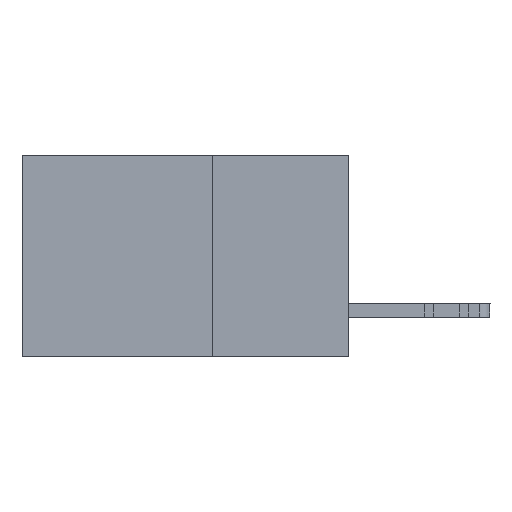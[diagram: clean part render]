
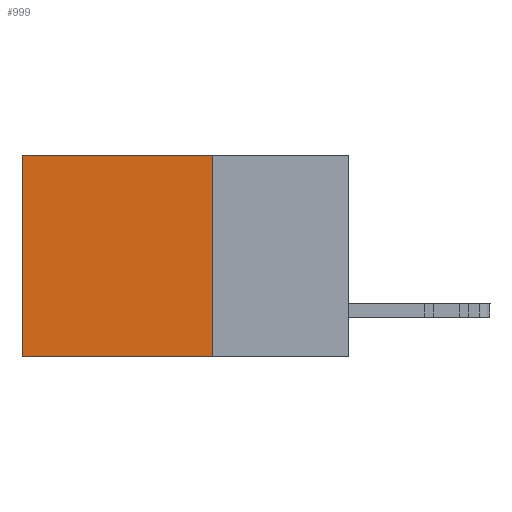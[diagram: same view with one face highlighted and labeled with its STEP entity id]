
A CAD part, left-side view. The second image highlights one B-rep face of the part: STEP entity #999.
In plain terms, the highlighted planar face has unit normal (-1, 0, 0).
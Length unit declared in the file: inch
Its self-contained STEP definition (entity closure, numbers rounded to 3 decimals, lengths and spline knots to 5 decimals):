
#294 = CARTESIAN_POINT ( 'NONE',  ( 0.2615, 0.25, -0.37 ) ) ;
#839 = DIRECTION ( 'NONE',  ( 0., 1., 0. ) ) ;
#999 = ADVANCED_FACE ( 'NONE', ( #12990 ), #22394, .F. ) ;
#1249 = VERTEX_POINT ( 'NONE', #13053 ) ;
#1746 = ORIENTED_EDGE ( 'NONE', *, *, #7309, .F. ) ;
#2405 = LINE ( 'NONE', #9855, #22892 ) ;
#4763 = CARTESIAN_POINT ( 'NONE',  ( 0.2615, 0.6, -0.37 ) ) ;
#5601 = VECTOR ( 'NONE', #7754, 39.37008 ) ;
#6305 = VERTEX_POINT ( 'NONE', #11732 ) ;
#7187 = CARTESIAN_POINT ( 'NONE',  ( 0.2615, 0.25, 0. ) ) ;
#7309 = EDGE_CURVE ( 'NONE', #17852, #19011, #2405, .T. ) ;
#7754 = DIRECTION ( 'NONE',  ( 0., 1., 0. ) ) ;
#8669 = AXIS2_PLACEMENT_3D ( 'NONE', #20450, #22514, #18620 ) ;
#9855 = CARTESIAN_POINT ( 'NONE',  ( 0.2615, 0.25, -0.37 ) ) ;
#10322 = ORIENTED_EDGE ( 'NONE', *, *, #18753, .F. ) ;
#11732 = CARTESIAN_POINT ( 'NONE',  ( 0.2615, 0.6, -0.37 ) ) ;
#11863 = VECTOR ( 'NONE', #12325, 39.37008 ) ;
#11963 = LINE ( 'NONE', #4763, #11863 ) ;
#12325 = DIRECTION ( 'NONE',  ( 0., 0., -1. ) ) ;
#12977 = EDGE_CURVE ( 'NONE', #17852, #1249, #16023, .T. ) ;
#12990 = FACE_OUTER_BOUND ( 'NONE', #19068, .T. ) ;
#13053 = CARTESIAN_POINT ( 'NONE',  ( 0.2615, 0.6, 0. ) ) ;
#13414 = ORIENTED_EDGE ( 'NONE', *, *, #19764, .T. ) ;
#14063 = CARTESIAN_POINT ( 'NONE',  ( 0.2615, 0.25, 0. ) ) ;
#16023 = LINE ( 'NONE', #14063, #16403 ) ;
#16403 = VECTOR ( 'NONE', #839, 39.37008 ) ;
#17324 = DIRECTION ( 'NONE',  ( 0., 0., -1. ) ) ;
#17852 = VERTEX_POINT ( 'NONE', #7187 ) ;
#18620 = DIRECTION ( 'NONE',  ( 0., 0., -1. ) ) ;
#18632 = CARTESIAN_POINT ( 'NONE',  ( 0.2615, 0.25, -0.37 ) ) ;
#18753 = EDGE_CURVE ( 'NONE', #19011, #6305, #19389, .T. ) ;
#19011 = VERTEX_POINT ( 'NONE', #18632 ) ;
#19068 = EDGE_LOOP ( 'NONE', ( #13414, #10322, #1746, #22504 ) ) ;
#19389 = LINE ( 'NONE', #294, #5601 ) ;
#19764 = EDGE_CURVE ( 'NONE', #1249, #6305, #11963, .T. ) ;
#20450 = CARTESIAN_POINT ( 'NONE',  ( 0.2615, 0.25, -0.37 ) ) ;
#22394 = PLANE ( 'NONE',  #8669 ) ;
#22504 = ORIENTED_EDGE ( 'NONE', *, *, #12977, .T. ) ;
#22514 = DIRECTION ( 'NONE',  ( 1., 0., 0. ) ) ;
#22892 = VECTOR ( 'NONE', #17324, 39.37008 ) ;
